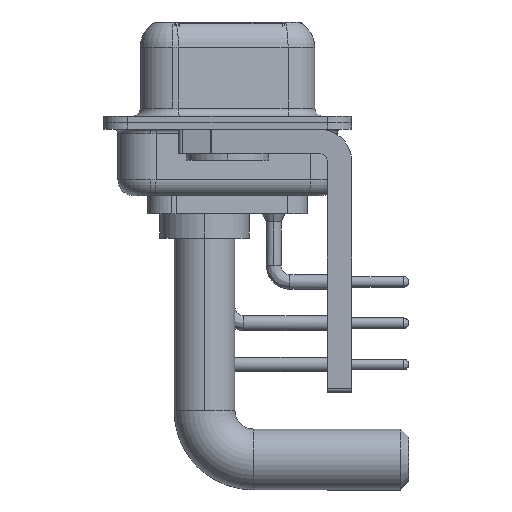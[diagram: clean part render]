
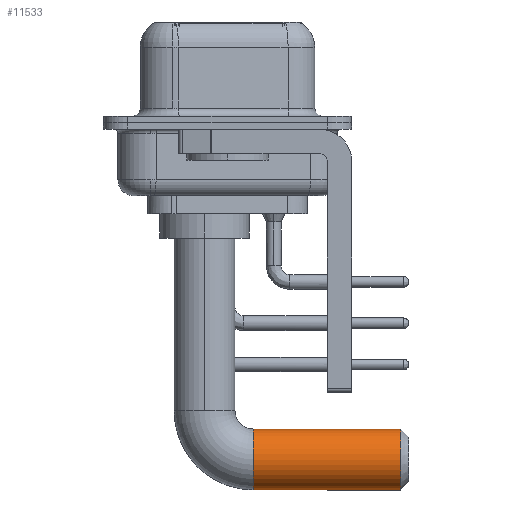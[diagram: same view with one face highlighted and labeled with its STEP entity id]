
A CAD part, left-side view. The second image highlights one B-rep face of the part: STEP entity #11533.
In plain terms, the highlighted cylindrical face has radius 1.875 mm (diameter 3.75 mm), a partial arc.
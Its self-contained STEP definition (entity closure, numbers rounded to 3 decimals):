
#1026 = CARTESIAN_POINT ( 'NONE',  ( 0., -12.07, -13.63 ) ) ;
#2028 = DIRECTION ( 'NONE',  ( -1., 0., 0. ) ) ;
#2463 = FACE_OUTER_BOUND ( 'NONE', #14012, .T. ) ;
#2498 = EDGE_CURVE ( 'NONE', #26945, #2897, #26102, .T. ) ;
#2632 = DIRECTION ( 'NONE',  ( 0., -1., 0. ) ) ;
#2897 = VERTEX_POINT ( 'NONE', #29704 ) ;
#3980 = CARTESIAN_POINT ( 'NONE',  ( 0., -3., -11.755 ) ) ;
#4981 = ORIENTED_EDGE ( 'NONE', *, *, #26636, .T. ) ;
#5053 = VECTOR ( 'NONE', #18840, 1000. ) ;
#8422 = DIRECTION ( 'NONE',  ( 0., -1., 0. ) ) ;
#9038 = CARTESIAN_POINT ( 'NONE',  ( 0., -3., -11.755 ) ) ;
#9738 = CIRCLE ( 'NONE', #22636, 1.875 ) ;
#11533 = ADVANCED_FACE ( 'NONE', ( #2463 ), #30410, .T. ) ;
#11580 = CARTESIAN_POINT ( 'NONE',  ( 0., -12.07, -11.755 ) ) ;
#11641 = CIRCLE ( 'NONE', #24550, 1.875 ) ;
#13949 = LINE ( 'NONE', #9038, #5053 ) ;
#14012 = EDGE_LOOP ( 'NONE', ( #26629, #4981, #18183, #27148 ) ) ;
#16261 = EDGE_CURVE ( 'NONE', #2897, #18437, #11641, .T. ) ;
#17639 = DIRECTION ( 'NONE',  ( 0., 0., -1. ) ) ;
#18183 = ORIENTED_EDGE ( 'NONE', *, *, #2498, .T. ) ;
#18437 = VERTEX_POINT ( 'NONE', #11580 ) ;
#18736 = DIRECTION ( 'NONE',  ( 0., 1., 0. ) ) ;
#18840 = DIRECTION ( 'NONE',  ( 0., -1., 0. ) ) ;
#19032 = CARTESIAN_POINT ( 'NONE',  ( 0., -3., -15.505 ) ) ;
#19378 = VECTOR ( 'NONE', #8422, 1000. ) ;
#22636 = AXIS2_PLACEMENT_3D ( 'NONE', #27790, #27627, #2028 ) ;
#22676 = CARTESIAN_POINT ( 'NONE',  ( 0., -3., -13.63 ) ) ;
#24550 = AXIS2_PLACEMENT_3D ( 'NONE', #1026, #18736, #29297 ) ;
#26102 = LINE ( 'NONE', #19032, #19378 ) ;
#26629 = ORIENTED_EDGE ( 'NONE', *, *, #32573, .F. ) ;
#26636 = EDGE_CURVE ( 'NONE', #32519, #26945, #9738, .T. ) ;
#26945 = VERTEX_POINT ( 'NONE', #31814 ) ;
#27148 = ORIENTED_EDGE ( 'NONE', *, *, #16261, .T. ) ;
#27627 = DIRECTION ( 'NONE',  ( 0., -1., 0. ) ) ;
#27790 = CARTESIAN_POINT ( 'NONE',  ( 0., -3., -13.63 ) ) ;
#29297 = DIRECTION ( 'NONE',  ( 0., 0., -1. ) ) ;
#29704 = CARTESIAN_POINT ( 'NONE',  ( 0., -12.07, -15.505 ) ) ;
#30259 = AXIS2_PLACEMENT_3D ( 'NONE', #22676, #2632, #17639 ) ;
#30410 = CYLINDRICAL_SURFACE ( 'NONE', #30259, 1.875 ) ;
#31814 = CARTESIAN_POINT ( 'NONE',  ( 0., -3., -15.505 ) ) ;
#32519 = VERTEX_POINT ( 'NONE', #3980 ) ;
#32573 = EDGE_CURVE ( 'NONE', #32519, #18437, #13949, .T. ) ;
